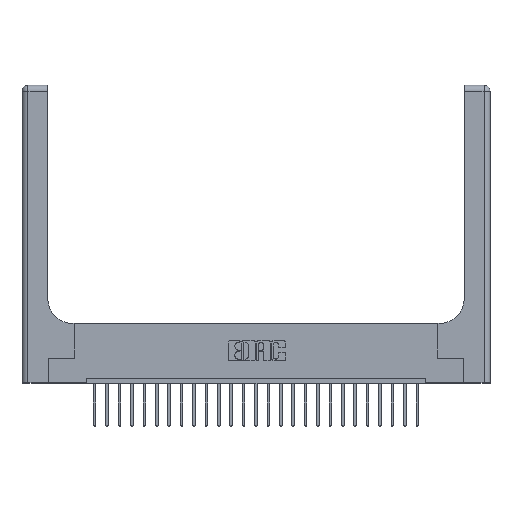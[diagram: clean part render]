
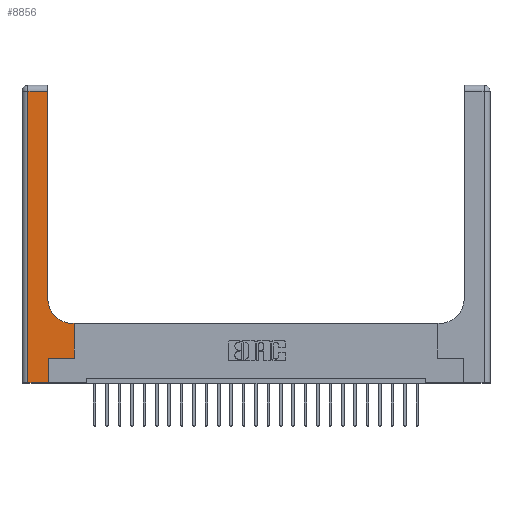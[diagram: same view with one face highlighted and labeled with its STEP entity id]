
A CAD part, top view. The second image highlights one B-rep face of the part: STEP entity #8856.
In plain terms, the highlighted planar face has unit normal (0, 0, 1).
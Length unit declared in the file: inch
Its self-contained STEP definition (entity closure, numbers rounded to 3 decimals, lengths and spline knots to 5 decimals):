
#3 = CARTESIAN_POINT ( 'NONE',  ( 0.51, 0.85, 0.37 ) ) ;
#454 = EDGE_CURVE ( 'NONE', #19969, #22612, #9355, .T. ) ;
#631 = VECTOR ( 'NONE', #11020, 39.37008 ) ;
#719 = CARTESIAN_POINT ( 'NONE',  ( 0.26, 0.85, 0.37 ) ) ;
#821 = VERTEX_POINT ( 'NONE', #22650 ) ;
#1194 = DIRECTION ( 'NONE',  ( 1., 0., 0. ) ) ;
#1280 = FACE_OUTER_BOUND ( 'NONE', #3637, .T. ) ;
#1517 = EDGE_CURVE ( 'NONE', #8996, #13830, #5507, .T. ) ;
#2283 = CARTESIAN_POINT ( 'NONE',  ( 0.265, 0., 0.37 ) ) ;
#2892 = CARTESIAN_POINT ( 'NONE',  ( 0.265, 0.25, 0.37 ) ) ;
#3172 = DIRECTION ( 'NONE',  ( 1., 0., 0. ) ) ;
#3408 = DIRECTION ( 'NONE',  ( 0., 1., 0. ) ) ;
#3637 = EDGE_LOOP ( 'NONE', ( #12215, #19871, #16823, #23544, #18374, #23054, #19663, #7515, #21277 ) ) ;
#4087 = CARTESIAN_POINT ( 'NONE',  ( 0., 2.94, 0.37 ) ) ;
#4152 = CARTESIAN_POINT ( 'NONE',  ( 0.265, 0., 0.37 ) ) ;
#4465 = VECTOR ( 'NONE', #4705, 39.37008 ) ;
#4705 = DIRECTION ( 'NONE',  ( -1., 0., 0. ) ) ;
#5159 = CARTESIAN_POINT ( 'NONE',  ( 0.26, 3., 0.37 ) ) ;
#5507 = LINE ( 'NONE', #18142, #631 ) ;
#5851 = VECTOR ( 'NONE', #17409, 39.37008 ) ;
#6056 = CARTESIAN_POINT ( 'NONE',  ( 0.528, 0.25, 0.37 ) ) ;
#7515 = ORIENTED_EDGE ( 'NONE', *, *, #8708, .T. ) ;
#7802 = EDGE_CURVE ( 'NONE', #7844, #20892, #16683, .T. ) ;
#7844 = VERTEX_POINT ( 'NONE', #19569 ) ;
#8341 = VECTOR ( 'NONE', #3408, 39.37008 ) ;
#8501 = CIRCLE ( 'NONE', #15254, 0.25 ) ;
#8506 = CARTESIAN_POINT ( 'NONE',  ( 0.528, 0.6, 0.37 ) ) ;
#8708 = EDGE_CURVE ( 'NONE', #13830, #821, #22711, .T. ) ;
#8754 = EDGE_CURVE ( 'NONE', #17374, #8996, #19778, .T. ) ;
#8856 = ADVANCED_FACE ( 'NONE', ( #1280 ), #16207, .F. ) ;
#8869 = EDGE_CURVE ( 'NONE', #821, #19674, #8501, .T. ) ;
#8938 = CARTESIAN_POINT ( 'NONE',  ( 0.26, 2.94, 0.37 ) ) ;
#8996 = VERTEX_POINT ( 'NONE', #6056 ) ;
#9355 = LINE ( 'NONE', #4087, #12509 ) ;
#9477 = EDGE_CURVE ( 'NONE', #20892, #17374, #12518, .T. ) ;
#10393 = DIRECTION ( 'NONE',  ( -1., 0., 0. ) ) ;
#10537 = DIRECTION ( 'NONE',  ( 0., 0., -1. ) ) ;
#10774 = DIRECTION ( 'NONE',  ( 0., 0., -1. ) ) ;
#11020 = DIRECTION ( 'NONE',  ( 0., 1., 0. ) ) ;
#11052 = VECTOR ( 'NONE', #11826, 39.37008 ) ;
#11826 = DIRECTION ( 'NONE',  ( 0., -1., 0. ) ) ;
#11997 = CARTESIAN_POINT ( 'NONE',  ( 0.26, 0.6, 0.37 ) ) ;
#12191 = EDGE_CURVE ( 'NONE', #19674, #19969, #21393, .T. ) ;
#12215 = ORIENTED_EDGE ( 'NONE', *, *, #12191, .T. ) ;
#12509 = VECTOR ( 'NONE', #10393, 39.37008 ) ;
#12518 = LINE ( 'NONE', #2283, #5851 ) ;
#13830 = VERTEX_POINT ( 'NONE', #8506 ) ;
#14308 = AXIS2_PLACEMENT_3D ( 'NONE', #17821, #10537, #21682 ) ;
#14593 = DIRECTION ( 'NONE',  ( 1., 0., 0. ) ) ;
#14844 = LINE ( 'NONE', #17284, #11052 ) ;
#15254 = AXIS2_PLACEMENT_3D ( 'NONE', #3, #10774, #14593 ) ;
#15578 = CARTESIAN_POINT ( 'NONE',  ( 0.06, 2.94, 0.37 ) ) ;
#15929 = CARTESIAN_POINT ( 'NONE',  ( 0., 0., 0.37 ) ) ;
#16207 = PLANE ( 'NONE',  #14308 ) ;
#16400 = VECTOR ( 'NONE', #1194, 39.37008 ) ;
#16683 = LINE ( 'NONE', #15929, #16400 ) ;
#16823 = ORIENTED_EDGE ( 'NONE', *, *, #22564, .T. ) ;
#17284 = CARTESIAN_POINT ( 'NONE',  ( 0.06, 3., 0.37 ) ) ;
#17374 = VERTEX_POINT ( 'NONE', #2892 ) ;
#17409 = DIRECTION ( 'NONE',  ( 0., 1., 0. ) ) ;
#17821 = CARTESIAN_POINT ( 'NONE',  ( 0., 3., 0.37 ) ) ;
#18142 = CARTESIAN_POINT ( 'NONE',  ( 0.528, 0.25, 0.37 ) ) ;
#18374 = ORIENTED_EDGE ( 'NONE', *, *, #9477, .T. ) ;
#18646 = VECTOR ( 'NONE', #3172, 39.37008 ) ;
#19569 = CARTESIAN_POINT ( 'NONE',  ( 0.06, 0., 0.37 ) ) ;
#19663 = ORIENTED_EDGE ( 'NONE', *, *, #1517, .T. ) ;
#19674 = VERTEX_POINT ( 'NONE', #719 ) ;
#19778 = LINE ( 'NONE', #23471, #18646 ) ;
#19871 = ORIENTED_EDGE ( 'NONE', *, *, #454, .T. ) ;
#19969 = VERTEX_POINT ( 'NONE', #8938 ) ;
#20892 = VERTEX_POINT ( 'NONE', #4152 ) ;
#21277 = ORIENTED_EDGE ( 'NONE', *, *, #8869, .T. ) ;
#21393 = LINE ( 'NONE', #5159, #8341 ) ;
#21682 = DIRECTION ( 'NONE',  ( -1., 0., 0. ) ) ;
#22564 = EDGE_CURVE ( 'NONE', #22612, #7844, #14844, .T. ) ;
#22612 = VERTEX_POINT ( 'NONE', #15578 ) ;
#22650 = CARTESIAN_POINT ( 'NONE',  ( 0.51, 0.6, 0.37 ) ) ;
#22711 = LINE ( 'NONE', #11997, #4465 ) ;
#23054 = ORIENTED_EDGE ( 'NONE', *, *, #8754, .T. ) ;
#23471 = CARTESIAN_POINT ( 'NONE',  ( 0.265, 0.25, 0.37 ) ) ;
#23544 = ORIENTED_EDGE ( 'NONE', *, *, #7802, .T. ) ;
